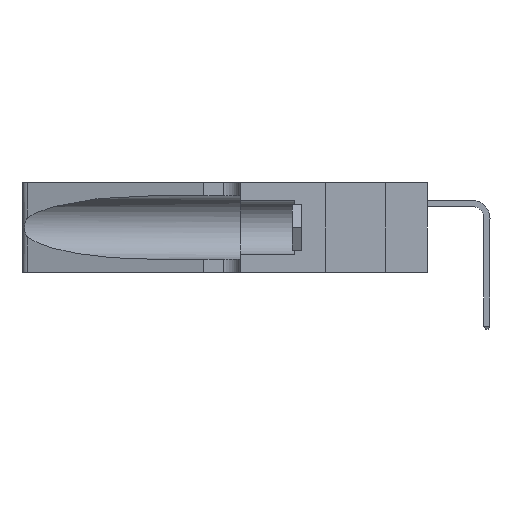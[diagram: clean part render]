
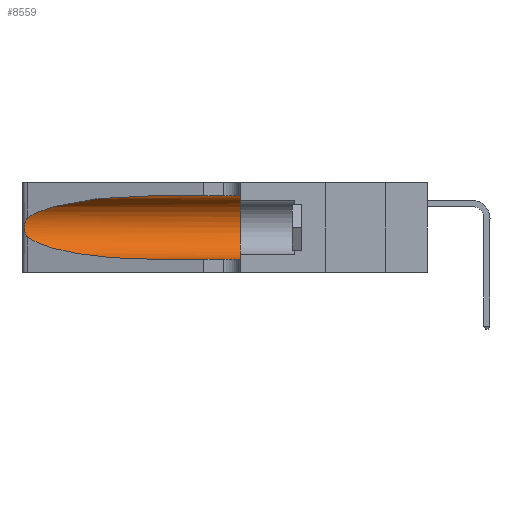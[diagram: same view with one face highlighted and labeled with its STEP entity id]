
A CAD part, left-side view. The second image highlights one B-rep face of the part: STEP entity #8559.
In plain terms, the highlighted cylindrical face has radius 3.308 mm (diameter 6.617 mm), a partial arc.
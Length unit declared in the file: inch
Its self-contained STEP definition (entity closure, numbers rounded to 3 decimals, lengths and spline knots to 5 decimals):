
#55 = CARTESIAN_POINT ( 'NONE',  ( 0.18966, 0.96281, 0.31525 ) ) ;
#499 = VECTOR ( 'NONE', #4461, 39.37008 ) ;
#1638 = CARTESIAN_POINT ( 'NONE',  ( 0.1305, 0.72297, 0.05475 ) ) ;
#1648 = DIRECTION ( 'NONE',  ( 0., 1., 0. ) ) ;
#1682 = EDGE_CURVE ( 'NONE', #5134, #31799, #9017, .T. ) ;
#2261 = CARTESIAN_POINT ( 'NONE',  ( 0.1305, 1.61858, 0.31525 ) ) ;
#2821 = CARTESIAN_POINT ( 'NONE',  ( 0.26075, 1.23896, 0.178 ) ) ;
#2915 = CARTESIAN_POINT ( 'NONE',  ( 0.1305, 0.72297, 0.31525 ) ) ;
#3058 = CARTESIAN_POINT ( 'NONE',  ( 0.25487, 1.22718, 0.14631 ) ) ;
#3746 = VERTEX_POINT ( 'NONE', #7704 ) ;
#3785 = EDGE_CURVE ( 'NONE', #3746, #5134, #8430, .T. ) ;
#4461 = DIRECTION ( 'NONE',  ( 0., -1., 0. ) ) ;
#5134 = VERTEX_POINT ( 'NONE', #11188 ) ;
#5663 = CARTESIAN_POINT ( 'NONE',  ( 0.25856, 1.23593, 0.16098 ) ) ;
#5751 = CARTESIAN_POINT ( 'NONE',  ( 0.2373, 1.15595, 0.28018 ) ) ;
#6696 = VECTOR ( 'NONE', #13446, 39.37008 ) ;
#6961 = FACE_OUTER_BOUND ( 'NONE', #27471, .T. ) ;
#7704 = CARTESIAN_POINT ( 'NONE',  ( 0.1305, 0.72297, 0.31525 ) ) ;
#8010 = CARTESIAN_POINT ( 'NONE',  ( 0.2373, 1.15595, 0.08982 ) ) ;
#8019 = LINE ( 'NONE', #12947, #499 ) ;
#8352 = CARTESIAN_POINT ( 'NONE',  ( 0.25487, 1.22718, 0.22369 ) ) ;
#8430 = LINE ( 'NONE', #2261, #6696 ) ;
#8480 = CARTESIAN_POINT ( 'NONE',  ( 0.25639, 1.23186, 0.15144 ) ) ;
#8559 = ADVANCED_FACE ( 'NONE', ( #6961 ), #20784, .F. ) ;
#9017 = CIRCLE ( 'NONE', #23534, 0.13025 ) ;
#10291 = ORIENTED_EDGE ( 'NONE', *, *, #29677, .T. ) ;
#10697 = VERTEX_POINT ( 'NONE', #1638 ) ;
#11073 = DIRECTION ( 'NONE',  ( 0., 0., -1. ) ) ;
#11188 = CARTESIAN_POINT ( 'NONE',  ( 0.1305, 0.35, 0.31525 ) ) ;
#11210 = CARTESIAN_POINT ( 'NONE',  ( 0.25487, 1.22718, 0.14631 ) ) ;
#12947 = CARTESIAN_POINT ( 'NONE',  ( 0.1305, 1.61858, 0.05475 ) ) ;
#13446 = DIRECTION ( 'NONE',  ( 0., -1., 0. ) ) ;
#13524 = CARTESIAN_POINT ( 'NONE',  ( 0.18966, 0.96281, 0.05475 ) ) ;
#13870 = CARTESIAN_POINT ( 'NONE',  ( 0.25639, 1.23184, 0.21858 ) ) ;
#14177 =( BOUNDED_CURVE ( )  B_SPLINE_CURVE ( 3, ( #27280, #8010, #13524, #32825 ),
 .UNSPECIFIED., .F., .F. ) 
 B_SPLINE_CURVE_WITH_KNOTS ( ( 4, 4 ),
 ( 3.44316, 4.71239 ),
 .UNSPECIFIED. ) 
 CURVE ( )  GEOMETRIC_REPRESENTATION_ITEM ( )  RATIONAL_B_SPLINE_CURVE ( ( 1., 0.87, 0.87, 1. ) ) 
 REPRESENTATION_ITEM ( '' )  );
#15434 =( BOUNDED_CURVE ( )  B_SPLINE_CURVE ( 3, ( #2915, #55, #5751, #25059 ),
 .UNSPECIFIED., .F., .F. ) 
 B_SPLINE_CURVE_WITH_KNOTS ( ( 4, 4 ),
 ( 1.5708, 2.84003 ),
 .UNSPECIFIED. ) 
 CURVE ( )  GEOMETRIC_REPRESENTATION_ITEM ( )  RATIONAL_B_SPLINE_CURVE ( ( 1., 0.87, 0.87, 1. ) ) 
 REPRESENTATION_ITEM ( '' )  );
#15987 = EDGE_CURVE ( 'NONE', #3746, #29372, #15434, .T. ) ;
#16283 = ORIENTED_EDGE ( 'NONE', *, *, #21742, .T. ) ;
#16612 = CARTESIAN_POINT ( 'NONE',  ( 0.1305, 1.61858, 0.185 ) ) ;
#16631 = CARTESIAN_POINT ( 'NONE',  ( 0.25854, 1.2359, 0.20912 ) ) ;
#18302 = CARTESIAN_POINT ( 'NONE',  ( 0.1305, 0.35, 0.185 ) ) ;
#19444 = CARTESIAN_POINT ( 'NONE',  ( 0.26075, 1.23896, 0.19203 ) ) ;
#20356 = CARTESIAN_POINT ( 'NONE',  ( 0.1305, 0.35, 0.05475 ) ) ;
#20784 = CYLINDRICAL_SURFACE ( 'NONE', #26429, 0.13025 ) ;
#20861 = EDGE_CURVE ( 'NONE', #10697, #31799, #8019, .T. ) ;
#21103 = DIRECTION ( 'NONE',  ( 0., 0., 1. ) ) ;
#21497 = ORIENTED_EDGE ( 'NONE', *, *, #15987, .T. ) ;
#21742 = EDGE_CURVE ( 'NONE', #29372, #25216, #22109, .T. ) ;
#22109 = B_SPLINE_CURVE_WITH_KNOTS ( 'NONE', 3,
 ( #8352, #30292, #13870, #33176, #16631, #26243, #19444, #2821, #22227, #5663, #24971, #8480, #27744, #11210 ),
 .UNSPECIFIED., .F., .F.,
 ( 4, 2, 2, 2, 2, 2, 4 ),
 ( 0., 0.00027, 0.00053, 0.00107, 0.0016, 0.00187, 0.00214 ),
 .UNSPECIFIED. ) ;
#22227 = CARTESIAN_POINT ( 'NONE',  ( 0.26017, 1.23833, 0.17102 ) ) ;
#23339 = CARTESIAN_POINT ( 'NONE',  ( 0.25487, 1.22718, 0.22369 ) ) ;
#23534 = AXIS2_PLACEMENT_3D ( 'NONE', #18302, #1648, #21103 ) ;
#24539 = ORIENTED_EDGE ( 'NONE', *, *, #20861, .T. ) ;
#24971 = CARTESIAN_POINT ( 'NONE',  ( 0.25789, 1.23486, 0.15765 ) ) ;
#25059 = CARTESIAN_POINT ( 'NONE',  ( 0.25487, 1.22718, 0.22369 ) ) ;
#25216 = VERTEX_POINT ( 'NONE', #3058 ) ;
#26243 = CARTESIAN_POINT ( 'NONE',  ( 0.26018, 1.23835, 0.19895 ) ) ;
#26429 = AXIS2_PLACEMENT_3D ( 'NONE', #16612, #35862, #11073 ) ;
#27280 = CARTESIAN_POINT ( 'NONE',  ( 0.25487, 1.22718, 0.14631 ) ) ;
#27471 = EDGE_LOOP ( 'NONE', ( #21497, #16283, #10291, #24539, #34607, #29487 ) ) ;
#27744 = CARTESIAN_POINT ( 'NONE',  ( 0.25555, 1.22993, 0.14849 ) ) ;
#29372 = VERTEX_POINT ( 'NONE', #23339 ) ;
#29487 = ORIENTED_EDGE ( 'NONE', *, *, #3785, .F. ) ;
#29677 = EDGE_CURVE ( 'NONE', #25216, #10697, #14177, .T. ) ;
#30292 = CARTESIAN_POINT ( 'NONE',  ( 0.25555, 1.22994, 0.2215 ) ) ;
#31799 = VERTEX_POINT ( 'NONE', #20356 ) ;
#32825 = CARTESIAN_POINT ( 'NONE',  ( 0.1305, 0.72297, 0.05475 ) ) ;
#33176 = CARTESIAN_POINT ( 'NONE',  ( 0.25787, 1.23484, 0.2124 ) ) ;
#34607 = ORIENTED_EDGE ( 'NONE', *, *, #1682, .F. ) ;
#35862 = DIRECTION ( 'NONE',  ( 0., -1., 0. ) ) ;
